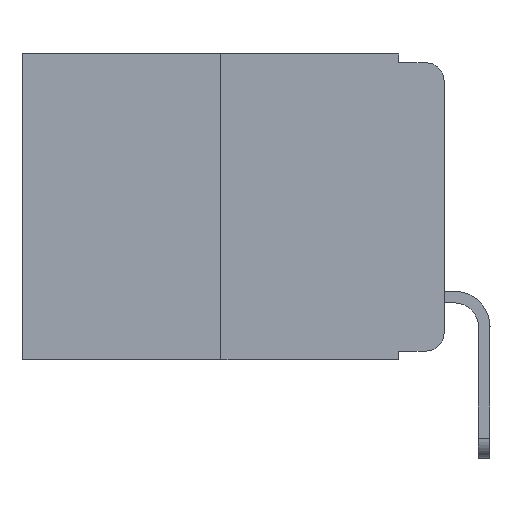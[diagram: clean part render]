
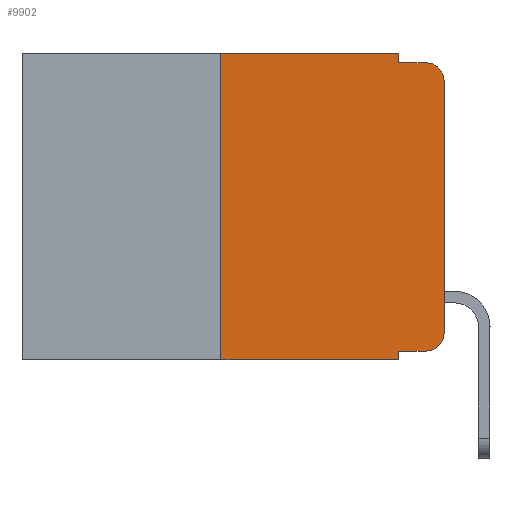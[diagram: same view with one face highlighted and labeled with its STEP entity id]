
A CAD part, left-side view. The second image highlights one B-rep face of the part: STEP entity #9902.
In plain terms, the highlighted planar face has unit normal (-1, 0, 0).
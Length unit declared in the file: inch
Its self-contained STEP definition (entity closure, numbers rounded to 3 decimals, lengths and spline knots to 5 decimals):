
#4 = EDGE_LOOP ( 'NONE', ( #1940, #13984, #76, #14995, #3035, #6134, #14405, #11874, #1856, #1016 ) ) ;
#38 = EDGE_CURVE ( 'NONE', #15749, #15521, #7221, .T. ) ;
#49 = VERTEX_POINT ( 'NONE', #12147 ) ;
#76 = ORIENTED_EDGE ( 'NONE', *, *, #2704, .F. ) ;
#405 = DIRECTION ( 'NONE',  ( 0., -1., 0. ) ) ;
#705 = DIRECTION ( 'NONE',  ( 0., -1., 0. ) ) ;
#861 = DIRECTION ( 'NONE',  ( 0., 0., -1. ) ) ;
#890 = CARTESIAN_POINT ( 'NONE',  ( 0., 0., 0. ) ) ;
#1016 = ORIENTED_EDGE ( 'NONE', *, *, #14107, .T. ) ;
#1021 = DIRECTION ( 'NONE',  ( 0., -1., 0. ) ) ;
#1342 = EDGE_CURVE ( 'NONE', #49, #8071, #14640, .T. ) ;
#1589 = EDGE_CURVE ( 'NONE', #6437, #7940, #5217, .T. ) ;
#1683 = DIRECTION ( 'NONE',  ( 0., 0., -1. ) ) ;
#1856 = ORIENTED_EDGE ( 'NONE', *, *, #5054, .T. ) ;
#1940 = ORIENTED_EDGE ( 'NONE', *, *, #38, .T. ) ;
#2006 = LINE ( 'NONE', #3288, #2232 ) ;
#2232 = VECTOR ( 'NONE', #705, 39.37008 ) ;
#2592 = EDGE_CURVE ( 'NONE', #8222, #4352, #11956, .T. ) ;
#2704 = EDGE_CURVE ( 'NONE', #4352, #15803, #9674, .T. ) ;
#2804 = CARTESIAN_POINT ( 'NONE',  ( 0., 0., -0.313 ) ) ;
#3035 = ORIENTED_EDGE ( 'NONE', *, *, #6761, .F. ) ;
#3288 = CARTESIAN_POINT ( 'NONE',  ( 0., 0.473, -0.343 ) ) ;
#3300 = DIRECTION ( 'NONE',  ( 0., -1., 0. ) ) ;
#3397 = CARTESIAN_POINT ( 'NONE',  ( 0., 0.051, 0. ) ) ;
#4352 = VERTEX_POINT ( 'NONE', #4487 ) ;
#4487 = CARTESIAN_POINT ( 'NONE',  ( 0., 0.051, -0.01 ) ) ;
#4519 = LINE ( 'NONE', #14426, #8447 ) ;
#4692 = CARTESIAN_POINT ( 'NONE',  ( 0., 0., -0.03 ) ) ;
#5054 = EDGE_CURVE ( 'NONE', #6437, #14747, #4519, .T. ) ;
#5217 = LINE ( 'NONE', #15038, #12006 ) ;
#5448 = CARTESIAN_POINT ( 'NONE',  ( 0., 0.473, 0. ) ) ;
#5608 = VECTOR ( 'NONE', #1021, 39.37008 ) ;
#5613 = PLANE ( 'NONE',  #13749 ) ;
#5724 = CIRCLE ( 'NONE', #6522, 0.02 ) ;
#6134 = ORIENTED_EDGE ( 'NONE', *, *, #1342, .F. ) ;
#6194 = DIRECTION ( 'NONE',  ( 0., 0., -1. ) ) ;
#6437 = VERTEX_POINT ( 'NONE', #7079 ) ;
#6522 = AXIS2_PLACEMENT_3D ( 'NONE', #16000, #15844, #6194 ) ;
#6761 = EDGE_CURVE ( 'NONE', #8071, #8222, #11576, .T. ) ;
#7002 = DIRECTION ( 'NONE',  ( 1., 0., 0. ) ) ;
#7079 = CARTESIAN_POINT ( 'NONE',  ( 0., 0.051, -0.333 ) ) ;
#7113 = CARTESIAN_POINT ( 'NONE',  ( 0., 0.25, 0. ) ) ;
#7221 = LINE ( 'NONE', #890, #12373 ) ;
#7364 = CIRCLE ( 'NONE', #7875, 0.02 ) ;
#7875 = AXIS2_PLACEMENT_3D ( 'NONE', #11410, #11731, #1683 ) ;
#7940 = VERTEX_POINT ( 'NONE', #8912 ) ;
#8071 = VERTEX_POINT ( 'NONE', #14105 ) ;
#8222 = VERTEX_POINT ( 'NONE', #3397 ) ;
#8447 = VECTOR ( 'NONE', #3300, 39.37008 ) ;
#8500 = DIRECTION ( 'NONE',  ( 0., 0., 1. ) ) ;
#8912 = CARTESIAN_POINT ( 'NONE',  ( 0., 0.051, -0.343 ) ) ;
#9202 = CARTESIAN_POINT ( 'NONE',  ( 0., 0.051, 0. ) ) ;
#9674 = LINE ( 'NONE', #14569, #5608 ) ;
#9902 = ADVANCED_FACE ( 'NONE', ( #13152 ), #5613, .F. ) ;
#9986 = DIRECTION ( 'NONE',  ( 0., 0., -1. ) ) ;
#10434 = CARTESIAN_POINT ( 'NONE',  ( 0., 0.473, 0. ) ) ;
#10539 = DIRECTION ( 'NONE',  ( 0., 0., -1. ) ) ;
#11323 = EDGE_CURVE ( 'NONE', #15521, #15803, #5724, .T. ) ;
#11410 = CARTESIAN_POINT ( 'NONE',  ( 0., 0.02, -0.313 ) ) ;
#11545 = VECTOR ( 'NONE', #861, 39.37008 ) ;
#11576 = LINE ( 'NONE', #10434, #13584 ) ;
#11717 = CARTESIAN_POINT ( 'NONE',  ( 0., 0.02, -0.01 ) ) ;
#11731 = DIRECTION ( 'NONE',  ( -1., 0., 0. ) ) ;
#11874 = ORIENTED_EDGE ( 'NONE', *, *, #1589, .F. ) ;
#11956 = LINE ( 'NONE', #9202, #11545 ) ;
#12006 = VECTOR ( 'NONE', #9986, 39.37008 ) ;
#12147 = CARTESIAN_POINT ( 'NONE',  ( 0., 0.25, -0.343 ) ) ;
#12373 = VECTOR ( 'NONE', #8500, 39.37008 ) ;
#13152 = FACE_OUTER_BOUND ( 'NONE', #4, .T. ) ;
#13584 = VECTOR ( 'NONE', #405, 39.37008 ) ;
#13749 = AXIS2_PLACEMENT_3D ( 'NONE', #5448, #7002, #10539 ) ;
#13984 = ORIENTED_EDGE ( 'NONE', *, *, #11323, .T. ) ;
#14105 = CARTESIAN_POINT ( 'NONE',  ( 0., 0.25, 0. ) ) ;
#14107 = EDGE_CURVE ( 'NONE', #14747, #15749, #7364, .T. ) ;
#14321 = VECTOR ( 'NONE', #15861, 39.37008 ) ;
#14405 = ORIENTED_EDGE ( 'NONE', *, *, #15854, .T. ) ;
#14426 = CARTESIAN_POINT ( 'NONE',  ( 0., 0.051, -0.333 ) ) ;
#14569 = CARTESIAN_POINT ( 'NONE',  ( 0., 0.051, -0.01 ) ) ;
#14640 = LINE ( 'NONE', #7113, #14321 ) ;
#14717 = CARTESIAN_POINT ( 'NONE',  ( 0., 0.02, -0.333 ) ) ;
#14747 = VERTEX_POINT ( 'NONE', #14717 ) ;
#14995 = ORIENTED_EDGE ( 'NONE', *, *, #2592, .F. ) ;
#15038 = CARTESIAN_POINT ( 'NONE',  ( 0., 0.051, 0. ) ) ;
#15521 = VERTEX_POINT ( 'NONE', #4692 ) ;
#15749 = VERTEX_POINT ( 'NONE', #2804 ) ;
#15803 = VERTEX_POINT ( 'NONE', #11717 ) ;
#15844 = DIRECTION ( 'NONE',  ( -1., 0., 0. ) ) ;
#15854 = EDGE_CURVE ( 'NONE', #49, #7940, #2006, .T. ) ;
#15861 = DIRECTION ( 'NONE',  ( 0., 0., 1. ) ) ;
#16000 = CARTESIAN_POINT ( 'NONE',  ( 0., 0.02, -0.03 ) ) ;
